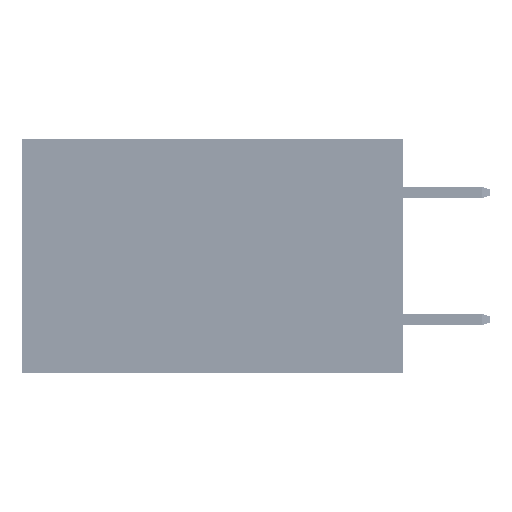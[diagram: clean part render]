
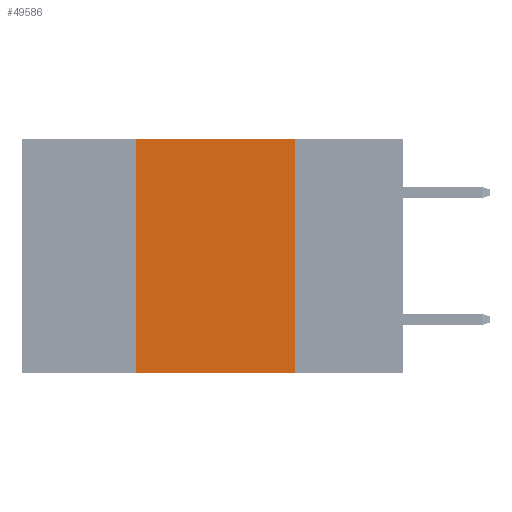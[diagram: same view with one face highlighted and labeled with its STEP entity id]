
A CAD part, left-side view. The second image highlights one B-rep face of the part: STEP entity #49586.
In plain terms, the highlighted planar face has unit normal (-1, 0, 0).
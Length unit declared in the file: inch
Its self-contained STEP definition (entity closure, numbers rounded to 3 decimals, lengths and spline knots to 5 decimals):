
#2658 = EDGE_LOOP ( 'NONE', ( #11591, #9996, #39149, #28155 ) ) ;
#5719 = LINE ( 'NONE', #14298, #18707 ) ;
#6321 = VERTEX_POINT ( 'NONE', #43427 ) ;
#8022 = CARTESIAN_POINT ( 'NONE',  ( 0., 0.6, 0. ) ) ;
#9056 = FACE_OUTER_BOUND ( 'NONE', #2658, .T. ) ;
#9875 = DIRECTION ( 'NONE',  ( 0., 0., 1. ) ) ;
#9996 = ORIENTED_EDGE ( 'NONE', *, *, #17788, .F. ) ;
#11591 = ORIENTED_EDGE ( 'NONE', *, *, #16484, .F. ) ;
#12169 = CARTESIAN_POINT ( 'NONE',  ( 0., 0.17, 0. ) ) ;
#12695 = DIRECTION ( 'NONE',  ( 0., 0., -1. ) ) ;
#14298 = CARTESIAN_POINT ( 'NONE',  ( 0., 0.42, 0. ) ) ;
#14316 = DIRECTION ( 'NONE',  ( 0., -1., 0. ) ) ;
#15808 = LINE ( 'NONE', #8022, #39528 ) ;
#16193 = EDGE_CURVE ( 'NONE', #29165, #6321, #5719, .T. ) ;
#16332 = CARTESIAN_POINT ( 'NONE',  ( 0., 0.6, 0. ) ) ;
#16484 = EDGE_CURVE ( 'NONE', #34441, #18565, #48260, .T. ) ;
#17788 = EDGE_CURVE ( 'NONE', #6321, #34441, #15808, .T. ) ;
#18565 = VERTEX_POINT ( 'NONE', #22460 ) ;
#18707 = VECTOR ( 'NONE', #9875, 39.37008 ) ;
#18711 = CARTESIAN_POINT ( 'NONE',  ( 0., 0.6, -0.37 ) ) ;
#22460 = CARTESIAN_POINT ( 'NONE',  ( 0., 0.17, -0.37 ) ) ;
#24907 = PLANE ( 'NONE',  #41916 ) ;
#28155 = ORIENTED_EDGE ( 'NONE', *, *, #43136, .T. ) ;
#29165 = VERTEX_POINT ( 'NONE', #37642 ) ;
#32676 = DIRECTION ( 'NONE',  ( 0., 0., -1. ) ) ;
#34441 = VERTEX_POINT ( 'NONE', #37696 ) ;
#37642 = CARTESIAN_POINT ( 'NONE',  ( 0., 0.42, -0.37 ) ) ;
#37696 = CARTESIAN_POINT ( 'NONE',  ( 0., 0.17, 0. ) ) ;
#39149 = ORIENTED_EDGE ( 'NONE', *, *, #16193, .F. ) ;
#39528 = VECTOR ( 'NONE', #50387, 39.37008 ) ;
#40286 = LINE ( 'NONE', #18711, #42407 ) ;
#40999 = DIRECTION ( 'NONE',  ( 1., 0., 0. ) ) ;
#41916 = AXIS2_PLACEMENT_3D ( 'NONE', #16332, #40999, #12695 ) ;
#42407 = VECTOR ( 'NONE', #14316, 39.37008 ) ;
#43136 = EDGE_CURVE ( 'NONE', #29165, #18565, #40286, .T. ) ;
#43427 = CARTESIAN_POINT ( 'NONE',  ( 0., 0.42, 0. ) ) ;
#45300 = VECTOR ( 'NONE', #32676, 39.37008 ) ;
#48260 = LINE ( 'NONE', #12169, #45300 ) ;
#49586 = ADVANCED_FACE ( 'NONE', ( #9056 ), #24907, .F. ) ;
#50387 = DIRECTION ( 'NONE',  ( 0., -1., 0. ) ) ;
